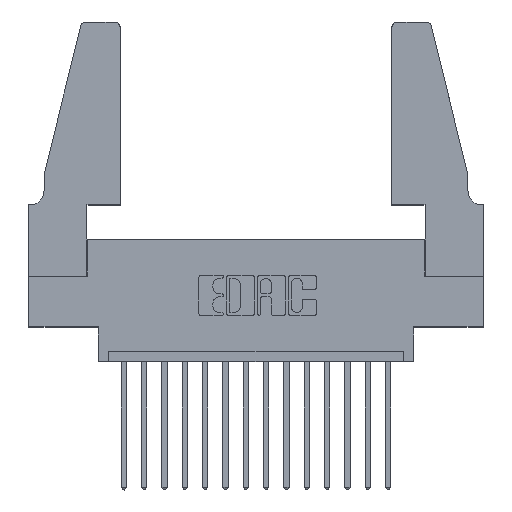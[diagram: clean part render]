
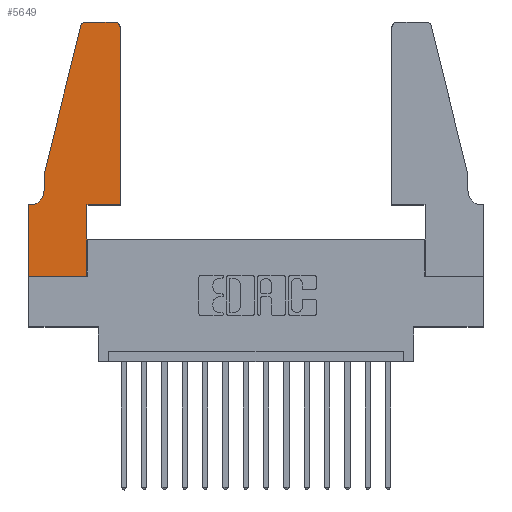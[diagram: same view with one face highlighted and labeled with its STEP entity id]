
A CAD part, top view. The second image highlights one B-rep face of the part: STEP entity #5649.
In plain terms, the highlighted planar face has unit normal (0, 0, 1).
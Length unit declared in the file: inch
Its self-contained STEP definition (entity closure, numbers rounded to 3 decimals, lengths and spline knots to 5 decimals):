
#24 = VECTOR ( 'NONE', #11651, 39.37008 ) ;
#132 = EDGE_CURVE ( 'NONE', #11721, #8921, #15669, .T. ) ;
#330 = EDGE_CURVE ( 'NONE', #6828, #11909, #598, .T. ) ;
#428 = EDGE_CURVE ( 'NONE', #13264, #14703, #13817, .T. ) ;
#430 = ORIENTED_EDGE ( 'NONE', *, *, #3171, .T. ) ;
#438 = VERTEX_POINT ( 'NONE', #6475 ) ;
#445 = EDGE_CURVE ( 'NONE', #9954, #3092, #3162, .T. ) ;
#598 = LINE ( 'NONE', #7142, #6181 ) ;
#809 = CIRCLE ( 'NONE', #14278, 0.03 ) ;
#953 = CARTESIAN_POINT ( 'NONE',  ( 0.0755, 0.5, 0.37 ) ) ;
#1004 = DIRECTION ( 'NONE',  ( 0., 0., 1. ) ) ;
#1087 = FACE_OUTER_BOUND ( 'NONE', #12301, .T. ) ;
#1595 = VECTOR ( 'NONE', #6076, 39.37008 ) ;
#2151 = CARTESIAN_POINT ( 'NONE',  ( 0.2865, 0., 0.37 ) ) ;
#2633 = ORIENTED_EDGE ( 'NONE', *, *, #428, .T. ) ;
#2687 = DIRECTION ( 'NONE',  ( -1., 0., 0. ) ) ;
#2712 = EDGE_CURVE ( 'NONE', #14703, #6828, #5026, .T. ) ;
#2764 = ORIENTED_EDGE ( 'NONE', *, *, #10580, .T. ) ;
#3092 = VERTEX_POINT ( 'NONE', #3520 ) ;
#3162 = LINE ( 'NONE', #11600, #24 ) ;
#3171 = EDGE_CURVE ( 'NONE', #10960, #9954, #6599, .T. ) ;
#3287 = AXIS2_PLACEMENT_3D ( 'NONE', #3604, #6006, #8580 ) ;
#3304 = LINE ( 'NONE', #14260, #6337 ) ;
#3520 = CARTESIAN_POINT ( 'NONE',  ( 0.4505, 1.22, 0.37 ) ) ;
#3521 = CARTESIAN_POINT ( 'NONE',  ( 0.4505, 0.35, 0.37 ) ) ;
#3604 = CARTESIAN_POINT ( 'NONE',  ( 0.4205, 1.22, 0.37 ) ) ;
#4081 = DIRECTION ( 'NONE',  ( 0., 0., 1. ) ) ;
#5026 = LINE ( 'NONE', #9154, #8416 ) ;
#5044 = AXIS2_PLACEMENT_3D ( 'NONE', #7712, #11419, #14217 ) ;
#5153 = CARTESIAN_POINT ( 'NONE',  ( 0.2605, 1.25, 0.37 ) ) ;
#5249 = EDGE_CURVE ( 'NONE', #11909, #13462, #3304, .T. ) ;
#5425 = VECTOR ( 'NONE', #13849, 39.37008 ) ;
#5494 = VERTEX_POINT ( 'NONE', #5980 ) ;
#5649 = ADVANCED_FACE ( 'NONE', ( #1087 ), #6095, .T. ) ;
#5980 = CARTESIAN_POINT ( 'NONE',  ( 0.284, 1.25, 0.37 ) ) ;
#6006 = DIRECTION ( 'NONE',  ( 0., 0., 1. ) ) ;
#6076 = DIRECTION ( 'NONE',  ( 1., 0., 0. ) ) ;
#6095 = PLANE ( 'NONE',  #14993 ) ;
#6181 = VECTOR ( 'NONE', #8431, 39.37008 ) ;
#6337 = VECTOR ( 'NONE', #13014, 39.37008 ) ;
#6475 = CARTESIAN_POINT ( 'NONE',  ( 0.4205, 1.25, 0.37 ) ) ;
#6575 = DIRECTION ( 'NONE',  ( 0., 1., 0. ) ) ;
#6599 = LINE ( 'NONE', #13169, #1595 ) ;
#6608 = VECTOR ( 'NONE', #2687, 39.37008 ) ;
#6758 = CARTESIAN_POINT ( 'NONE',  ( 0.284, 1.22, 0.37 ) ) ;
#6776 = VECTOR ( 'NONE', #6575, 39.37008 ) ;
#6828 = VERTEX_POINT ( 'NONE', #9530 ) ;
#6978 = DIRECTION ( 'NONE',  ( -0.239, -0.971, 0. ) ) ;
#7064 = CARTESIAN_POINT ( 'NONE',  ( 0.0755, 0.5, 0.37 ) ) ;
#7129 = ORIENTED_EDGE ( 'NONE', *, *, #10211, .T. ) ;
#7142 = CARTESIAN_POINT ( 'NONE',  ( 0., 0., 0.37 ) ) ;
#7396 = CARTESIAN_POINT ( 'NONE',  ( 0., 0.35, 0.37 ) ) ;
#7445 = LINE ( 'NONE', #953, #5425 ) ;
#7575 = CARTESIAN_POINT ( 'NONE',  ( 0.0055, 0.35, 0.37 ) ) ;
#7712 = CARTESIAN_POINT ( 'NONE',  ( 0.0055, 0.42, 0.37 ) ) ;
#8180 = LINE ( 'NONE', #12897, #6776 ) ;
#8416 = VECTOR ( 'NONE', #15628, 39.37008 ) ;
#8431 = DIRECTION ( 'NONE',  ( 0., -1., 0. ) ) ;
#8580 = DIRECTION ( 'NONE',  ( 1., 0., 0. ) ) ;
#8646 = ORIENTED_EDGE ( 'NONE', *, *, #16228, .T. ) ;
#8921 = VERTEX_POINT ( 'NONE', #7064 ) ;
#9058 = CARTESIAN_POINT ( 'NONE',  ( 0.2865, 0.35, 0.37 ) ) ;
#9154 = CARTESIAN_POINT ( 'NONE',  ( 0.0755, 0.35, 0.37 ) ) ;
#9355 = DIRECTION ( 'NONE',  ( 1., 0., 0. ) ) ;
#9530 = CARTESIAN_POINT ( 'NONE',  ( 0., 0.35, 0.37 ) ) ;
#9558 = ORIENTED_EDGE ( 'NONE', *, *, #330, .T. ) ;
#9791 = ORIENTED_EDGE ( 'NONE', *, *, #445, .T. ) ;
#9876 = ORIENTED_EDGE ( 'NONE', *, *, #9910, .T. ) ;
#9910 = EDGE_CURVE ( 'NONE', #8921, #13264, #7445, .T. ) ;
#9954 = VERTEX_POINT ( 'NONE', #3521 ) ;
#10211 = EDGE_CURVE ( 'NONE', #3092, #438, #15701, .T. ) ;
#10367 = ORIENTED_EDGE ( 'NONE', *, *, #2712, .T. ) ;
#10580 = EDGE_CURVE ( 'NONE', #5494, #11721, #809, .T. ) ;
#10836 = LINE ( 'NONE', #5153, #6608 ) ;
#10960 = VERTEX_POINT ( 'NONE', #9058 ) ;
#11419 = DIRECTION ( 'NONE',  ( 0., 0., -1. ) ) ;
#11600 = CARTESIAN_POINT ( 'NONE',  ( 0.4505, 0.35, 0.37 ) ) ;
#11651 = DIRECTION ( 'NONE',  ( 0., 1., 0. ) ) ;
#11703 = EDGE_CURVE ( 'NONE', #438, #5494, #10836, .T. ) ;
#11721 = VERTEX_POINT ( 'NONE', #11722 ) ;
#11722 = CARTESIAN_POINT ( 'NONE',  ( 0.25487, 1.22718, 0.37 ) ) ;
#11761 = ORIENTED_EDGE ( 'NONE', *, *, #5249, .T. ) ;
#11909 = VERTEX_POINT ( 'NONE', #12857 ) ;
#11925 = CARTESIAN_POINT ( 'NONE',  ( 0.0755, 0.42, 0.37 ) ) ;
#12301 = EDGE_LOOP ( 'NONE', ( #15453, #2764, #14587, #9876, #2633, #10367, #9558, #11761, #8646, #430, #9791, #7129 ) ) ;
#12857 = CARTESIAN_POINT ( 'NONE',  ( 0., 0., 0.37 ) ) ;
#12897 = CARTESIAN_POINT ( 'NONE',  ( 0.2865, 0.35, 0.37 ) ) ;
#13014 = DIRECTION ( 'NONE',  ( 1., 0., 0. ) ) ;
#13169 = CARTESIAN_POINT ( 'NONE',  ( 0.4505, 0.35, 0.37 ) ) ;
#13264 = VERTEX_POINT ( 'NONE', #11925 ) ;
#13375 = CARTESIAN_POINT ( 'NONE',  ( 0.0755, 0.5, 0.37 ) ) ;
#13462 = VERTEX_POINT ( 'NONE', #2151 ) ;
#13817 = CIRCLE ( 'NONE', #5044, 0.07 ) ;
#13849 = DIRECTION ( 'NONE',  ( 0., -1., 0. ) ) ;
#14217 = DIRECTION ( 'NONE',  ( -1., 0., 0. ) ) ;
#14260 = CARTESIAN_POINT ( 'NONE',  ( 0., 0., 0.37 ) ) ;
#14278 = AXIS2_PLACEMENT_3D ( 'NONE', #6758, #4081, #9355 ) ;
#14587 = ORIENTED_EDGE ( 'NONE', *, *, #132, .T. ) ;
#14703 = VERTEX_POINT ( 'NONE', #7575 ) ;
#14835 = VECTOR ( 'NONE', #6978, 39.37008 ) ;
#14993 = AXIS2_PLACEMENT_3D ( 'NONE', #7396, #1004, #15161 ) ;
#15161 = DIRECTION ( 'NONE',  ( 1., 0., 0. ) ) ;
#15453 = ORIENTED_EDGE ( 'NONE', *, *, #11703, .T. ) ;
#15628 = DIRECTION ( 'NONE',  ( -1., 0., 0. ) ) ;
#15669 = LINE ( 'NONE', #13375, #14835 ) ;
#15701 = CIRCLE ( 'NONE', #3287, 0.03 ) ;
#16228 = EDGE_CURVE ( 'NONE', #13462, #10960, #8180, .T. ) ;
